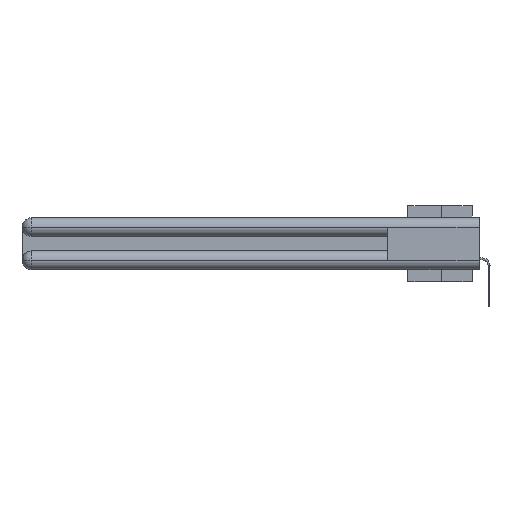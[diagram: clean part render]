
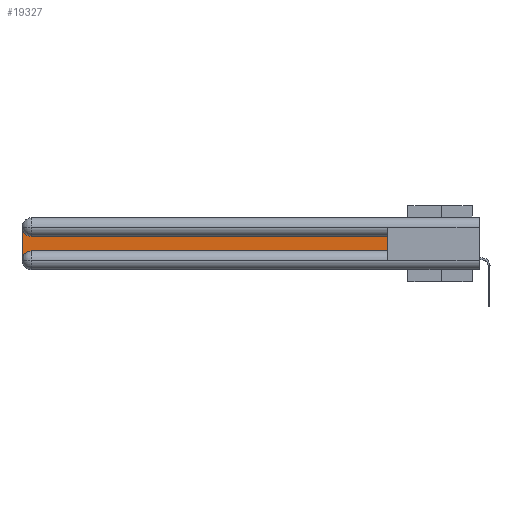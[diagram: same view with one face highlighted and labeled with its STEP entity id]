
A CAD part, left-side view. The second image highlights one B-rep face of the part: STEP entity #19327.
In plain terms, the highlighted planar face has unit normal (-1, 0, 0).
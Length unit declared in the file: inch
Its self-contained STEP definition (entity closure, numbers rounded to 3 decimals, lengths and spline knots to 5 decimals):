
#1123 = VECTOR ( 'NONE', #20282, 39.37008 ) ;
#1587 = CARTESIAN_POINT ( 'NONE',  ( 0.075, 0.6, -0.2175 ) ) ;
#1742 = VERTEX_POINT ( 'NONE', #27883 ) ;
#2463 = CARTESIAN_POINT ( 'NONE',  ( 0.075, 3., -0.0625 ) ) ;
#3252 = DIRECTION ( 'NONE',  ( 1., 0., 0. ) ) ;
#3494 = VERTEX_POINT ( 'NONE', #14694 ) ;
#3639 = VECTOR ( 'NONE', #4675, 39.37008 ) ;
#4675 = DIRECTION ( 'NONE',  ( 0., 1., 0. ) ) ;
#5235 = CARTESIAN_POINT ( 'NONE',  ( 0.075, 0.6, -0.1225 ) ) ;
#6940 = DIRECTION ( 'NONE',  ( 0., 0., -1. ) ) ;
#7254 = VECTOR ( 'NONE', #16224, 39.37008 ) ;
#7346 = AXIS2_PLACEMENT_3D ( 'NONE', #16760, #14908, #6940 ) ;
#9095 = CARTESIAN_POINT ( 'NONE',  ( 0.075, 0.6, -0.2175 ) ) ;
#9154 = EDGE_CURVE ( 'NONE', #3494, #1742, #25776, .T. ) ;
#10875 = LINE ( 'NONE', #11407, #7254 ) ;
#11407 = CARTESIAN_POINT ( 'NONE',  ( 0.075, 0.6, -0.2175 ) ) ;
#12068 = FACE_OUTER_BOUND ( 'NONE', #16714, .T. ) ;
#12857 = ORIENTED_EDGE ( 'NONE', *, *, #33828, .T. ) ;
#13570 = VECTOR ( 'NONE', #32677, 39.37008 ) ;
#14694 = CARTESIAN_POINT ( 'NONE',  ( 0.075, 3., -0.2775 ) ) ;
#14908 = DIRECTION ( 'NONE',  ( 1., 0., 0. ) ) ;
#16224 = DIRECTION ( 'NONE',  ( 0., 0., 1. ) ) ;
#16352 = DIRECTION ( 'NONE',  ( 0., 0., -1. ) ) ;
#16714 = EDGE_LOOP ( 'NONE', ( #28235, #12857, #33250, #29785, #33649, #19855 ) ) ;
#16760 = CARTESIAN_POINT ( 'NONE',  ( 0.075, 3., -0.1225 ) ) ;
#17117 = DIRECTION ( 'NONE',  ( 1., 0., 0. ) ) ;
#17490 = EDGE_CURVE ( 'NONE', #1742, #32715, #22773, .T. ) ;
#17746 = EDGE_CURVE ( 'NONE', #34926, #3494, #29666, .T. ) ;
#17819 = CIRCLE ( 'NONE', #25766, 0.06 ) ;
#19327 = ADVANCED_FACE ( 'NONE', ( #12068 ), #22932, .F. ) ;
#19358 = CARTESIAN_POINT ( 'NONE',  ( 0.075, 3., -0.2175 ) ) ;
#19855 = ORIENTED_EDGE ( 'NONE', *, *, #23187, .T. ) ;
#20282 = DIRECTION ( 'NONE',  ( 0., -1., 0. ) ) ;
#21182 = LINE ( 'NONE', #31845, #3639 ) ;
#22183 = VERTEX_POINT ( 'NONE', #5235 ) ;
#22461 = CARTESIAN_POINT ( 'NONE',  ( 0.075, 2.94, -0.2775 ) ) ;
#22773 = LINE ( 'NONE', #9095, #1123 ) ;
#22932 = PLANE ( 'NONE',  #7346 ) ;
#23187 = EDGE_CURVE ( 'NONE', #32715, #22183, #10875, .T. ) ;
#25766 = AXIS2_PLACEMENT_3D ( 'NONE', #29696, #3252, #16352 ) ;
#25776 = CIRCLE ( 'NONE', #28607, 0.06 ) ;
#27883 = CARTESIAN_POINT ( 'NONE',  ( 0.075, 2.94, -0.2175 ) ) ;
#27944 = DIRECTION ( 'NONE',  ( 0., 0., -1. ) ) ;
#28235 = ORIENTED_EDGE ( 'NONE', *, *, #29462, .T. ) ;
#28607 = AXIS2_PLACEMENT_3D ( 'NONE', #22461, #17117, #27944 ) ;
#28841 = VERTEX_POINT ( 'NONE', #34196 ) ;
#29462 = EDGE_CURVE ( 'NONE', #22183, #28841, #21182, .T. ) ;
#29666 = LINE ( 'NONE', #19358, #13570 ) ;
#29696 = CARTESIAN_POINT ( 'NONE',  ( 0.075, 2.94, -0.0625 ) ) ;
#29785 = ORIENTED_EDGE ( 'NONE', *, *, #9154, .T. ) ;
#31845 = CARTESIAN_POINT ( 'NONE',  ( 0.075, 0.6, -0.1225 ) ) ;
#32677 = DIRECTION ( 'NONE',  ( 0., 0., -1. ) ) ;
#32715 = VERTEX_POINT ( 'NONE', #1587 ) ;
#33250 = ORIENTED_EDGE ( 'NONE', *, *, #17746, .T. ) ;
#33649 = ORIENTED_EDGE ( 'NONE', *, *, #17490, .T. ) ;
#33828 = EDGE_CURVE ( 'NONE', #28841, #34926, #17819, .T. ) ;
#34196 = CARTESIAN_POINT ( 'NONE',  ( 0.075, 2.94, -0.1225 ) ) ;
#34926 = VERTEX_POINT ( 'NONE', #2463 ) ;
